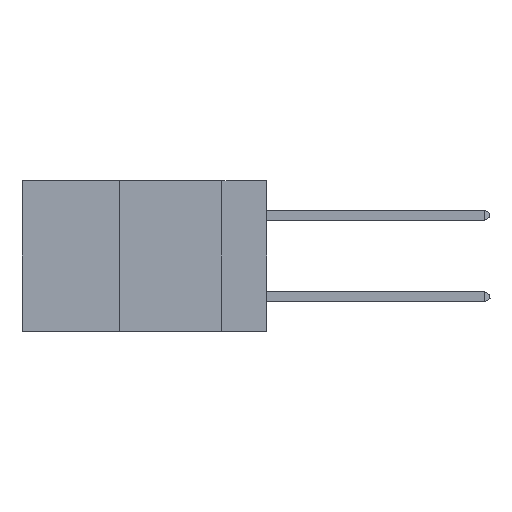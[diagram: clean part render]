
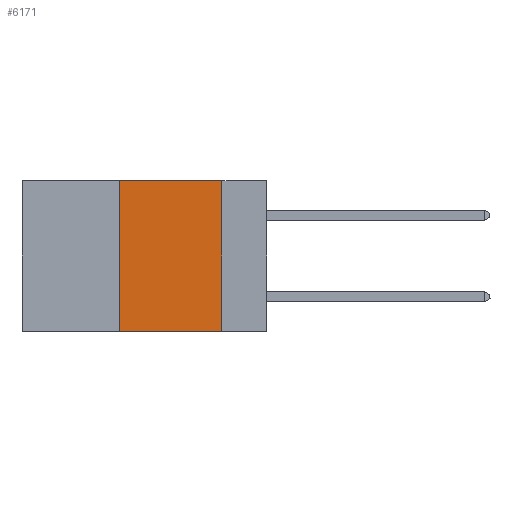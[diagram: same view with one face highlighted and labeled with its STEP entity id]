
A CAD part, left-side view. The second image highlights one B-rep face of the part: STEP entity #6171.
In plain terms, the highlighted planar face has unit normal (-1, 0, 0).
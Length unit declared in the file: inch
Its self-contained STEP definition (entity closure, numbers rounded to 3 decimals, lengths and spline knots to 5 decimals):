
#11 = FACE_OUTER_BOUND ( 'NONE', #4279, .T. ) ;
#37 = EDGE_CURVE ( 'NONE', #12401, #33352, #38135, .T. ) ;
#3468 = ORIENTED_EDGE ( 'NONE', *, *, #37, .T. ) ;
#4279 = EDGE_LOOP ( 'NONE', ( #24632, #22478, #5072, #3468 ) ) ;
#5072 = ORIENTED_EDGE ( 'NONE', *, *, #26016, .F. ) ;
#6171 = ADVANCED_FACE ( 'NONE', ( #11 ), #17200, .F. ) ;
#6179 = VECTOR ( 'NONE', #19718, 39.37008 ) ;
#6944 = CARTESIAN_POINT ( 'NONE',  ( 0., 0.11, -0.37 ) ) ;
#7120 = AXIS2_PLACEMENT_3D ( 'NONE', #40286, #14480, #20528 ) ;
#9735 = VECTOR ( 'NONE', #39557, 39.37008 ) ;
#9809 = VERTEX_POINT ( 'NONE', #16693 ) ;
#12401 = VERTEX_POINT ( 'NONE', #26123 ) ;
#13648 = CARTESIAN_POINT ( 'NONE',  ( 0., 0.11, 0. ) ) ;
#14480 = DIRECTION ( 'NONE',  ( 1., 0., 0. ) ) ;
#16464 = LINE ( 'NONE', #13648, #30389 ) ;
#16514 = EDGE_CURVE ( 'NONE', #34480, #33352, #16464, .T. ) ;
#16693 = CARTESIAN_POINT ( 'NONE',  ( 0., 0.36, 0. ) ) ;
#17200 = PLANE ( 'NONE',  #7120 ) ;
#17727 = CARTESIAN_POINT ( 'NONE',  ( 0., 0.36, 0. ) ) ;
#19718 = DIRECTION ( 'NONE',  ( 0., -1., 0. ) ) ;
#20528 = DIRECTION ( 'NONE',  ( 0., 0., -1. ) ) ;
#20897 = DIRECTION ( 'NONE',  ( 0., 0., 1. ) ) ;
#22478 = ORIENTED_EDGE ( 'NONE', *, *, #37066, .F. ) ;
#24632 = ORIENTED_EDGE ( 'NONE', *, *, #16514, .F. ) ;
#26016 = EDGE_CURVE ( 'NONE', #12401, #9809, #36847, .T. ) ;
#26123 = CARTESIAN_POINT ( 'NONE',  ( 0., 0.36, -0.37 ) ) ;
#26280 = CARTESIAN_POINT ( 'NONE',  ( 0., 0.6, -0.37 ) ) ;
#27328 = DIRECTION ( 'NONE',  ( 0., 0., -1. ) ) ;
#28098 = VECTOR ( 'NONE', #20897, 39.37008 ) ;
#30389 = VECTOR ( 'NONE', #27328, 39.37008 ) ;
#33352 = VERTEX_POINT ( 'NONE', #6944 ) ;
#34480 = VERTEX_POINT ( 'NONE', #36175 ) ;
#36144 = CARTESIAN_POINT ( 'NONE',  ( 0., 0.6, 0. ) ) ;
#36175 = CARTESIAN_POINT ( 'NONE',  ( 0., 0.11, 0. ) ) ;
#36656 = LINE ( 'NONE', #36144, #6179 ) ;
#36847 = LINE ( 'NONE', #17727, #28098 ) ;
#37066 = EDGE_CURVE ( 'NONE', #9809, #34480, #36656, .T. ) ;
#38135 = LINE ( 'NONE', #26280, #9735 ) ;
#39557 = DIRECTION ( 'NONE',  ( 0., -1., 0. ) ) ;
#40286 = CARTESIAN_POINT ( 'NONE',  ( 0., 0.6, 0. ) ) ;
